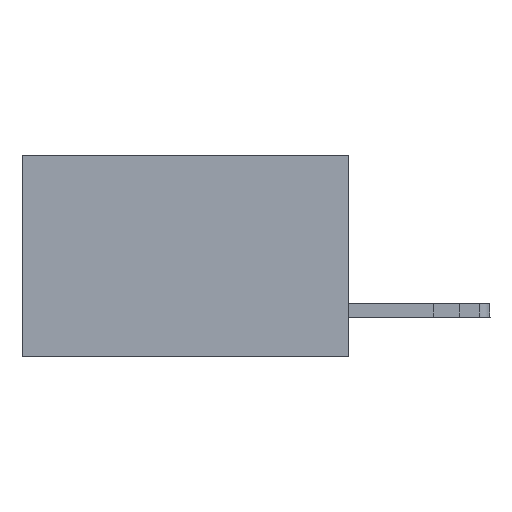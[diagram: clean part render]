
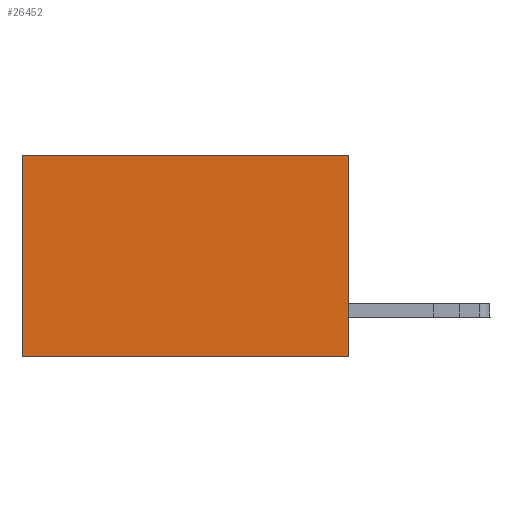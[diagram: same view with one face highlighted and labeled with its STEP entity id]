
A CAD part, left-side view. The second image highlights one B-rep face of the part: STEP entity #26452.
In plain terms, the highlighted planar face has unit normal (-1, 0, 0).
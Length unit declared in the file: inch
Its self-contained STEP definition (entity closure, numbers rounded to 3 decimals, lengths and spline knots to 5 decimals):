
#1097 = VERTEX_POINT ( 'NONE', #12435 ) ;
#1933 = VECTOR ( 'NONE', #17096, 39.37008 ) ;
#2055 = DIRECTION ( 'NONE',  ( 0., 0., -1. ) ) ;
#2551 = VECTOR ( 'NONE', #2055, 39.37008 ) ;
#3136 = CARTESIAN_POINT ( 'NONE',  ( 0.298, 0.6, 0. ) ) ;
#3610 = FACE_OUTER_BOUND ( 'NONE', #4194, .T. ) ;
#3742 = DIRECTION ( 'NONE',  ( 0., 0., -1. ) ) ;
#3997 = VECTOR ( 'NONE', #5323, 39.37008 ) ;
#4194 = EDGE_LOOP ( 'NONE', ( #8607, #18658, #20882, #15420 ) ) ;
#5323 = DIRECTION ( 'NONE',  ( 0., 0., -1. ) ) ;
#6117 = CARTESIAN_POINT ( 'NONE',  ( 0.298, 0., 0. ) ) ;
#6411 = LINE ( 'NONE', #8245, #2551 ) ;
#8245 = CARTESIAN_POINT ( 'NONE',  ( 0.298, 0.6, 0. ) ) ;
#8607 = ORIENTED_EDGE ( 'NONE', *, *, #9493, .T. ) ;
#8617 = CARTESIAN_POINT ( 'NONE',  ( 0.298, 0., -0.37 ) ) ;
#9117 = VECTOR ( 'NONE', #20200, 39.37008 ) ;
#9493 = EDGE_CURVE ( 'NONE', #14806, #1097, #6411, .T. ) ;
#9525 = CARTESIAN_POINT ( 'NONE',  ( 0.298, 0., 0. ) ) ;
#10209 = DIRECTION ( 'NONE',  ( 1., 0., 0. ) ) ;
#10784 = CARTESIAN_POINT ( 'NONE',  ( 0.298, 0., -0.37 ) ) ;
#11370 = CARTESIAN_POINT ( 'NONE',  ( 0.298, 0., 0. ) ) ;
#11407 = EDGE_CURVE ( 'NONE', #26459, #12070, #26564, .T. ) ;
#12070 = VERTEX_POINT ( 'NONE', #8617 ) ;
#12435 = CARTESIAN_POINT ( 'NONE',  ( 0.298, 0.6, -0.37 ) ) ;
#14806 = VERTEX_POINT ( 'NONE', #3136 ) ;
#15420 = ORIENTED_EDGE ( 'NONE', *, *, #18341, .T. ) ;
#17096 = DIRECTION ( 'NONE',  ( 0., 1., 0. ) ) ;
#18341 = EDGE_CURVE ( 'NONE', #26459, #14806, #22330, .T. ) ;
#18658 = ORIENTED_EDGE ( 'NONE', *, *, #18812, .F. ) ;
#18812 = EDGE_CURVE ( 'NONE', #12070, #1097, #25285, .T. ) ;
#20200 = DIRECTION ( 'NONE',  ( 0., 1., 0. ) ) ;
#20882 = ORIENTED_EDGE ( 'NONE', *, *, #11407, .F. ) ;
#20887 = AXIS2_PLACEMENT_3D ( 'NONE', #23418, #10209, #3742 ) ;
#22330 = LINE ( 'NONE', #9525, #9117 ) ;
#23418 = CARTESIAN_POINT ( 'NONE',  ( 0.298, 0., 0. ) ) ;
#25119 = PLANE ( 'NONE',  #20887 ) ;
#25285 = LINE ( 'NONE', #10784, #1933 ) ;
#26452 = ADVANCED_FACE ( 'NONE', ( #3610 ), #25119, .F. ) ;
#26459 = VERTEX_POINT ( 'NONE', #6117 ) ;
#26564 = LINE ( 'NONE', #11370, #3997 ) ;
